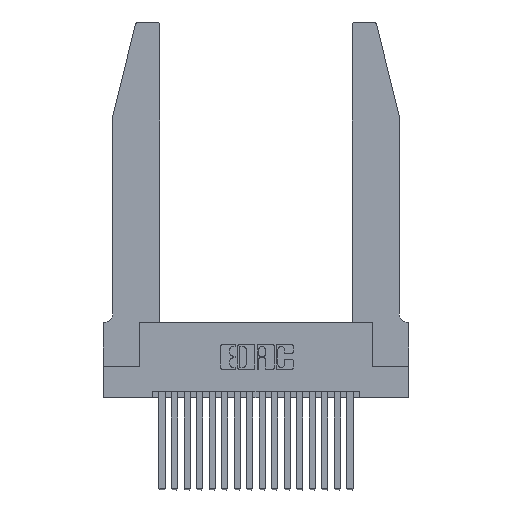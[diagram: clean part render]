
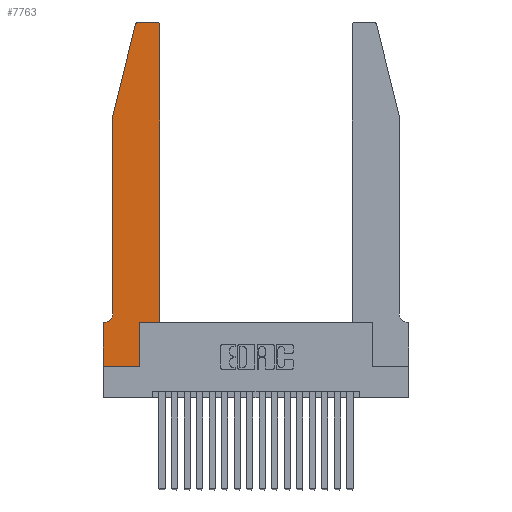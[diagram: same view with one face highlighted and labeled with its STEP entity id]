
A CAD part, top view. The second image highlights one B-rep face of the part: STEP entity #7763.
In plain terms, the highlighted planar face has unit normal (0, 0, 1).
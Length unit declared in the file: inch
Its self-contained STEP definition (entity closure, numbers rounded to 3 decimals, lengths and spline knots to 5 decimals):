
#69 = DIRECTION ( 'NONE',  ( 0., 1., 0. ) ) ;
#285 = ORIENTED_EDGE ( 'NONE', *, *, #6838, .T. ) ;
#444 = DIRECTION ( 'NONE',  ( 1., 0., 0. ) ) ;
#579 = CARTESIAN_POINT ( 'NONE',  ( 0.0755, 2., 0.37 ) ) ;
#1113 = VERTEX_POINT ( 'NONE', #9203 ) ;
#1130 = LINE ( 'NONE', #14866, #9741 ) ;
#1333 = CARTESIAN_POINT ( 'NONE',  ( 0., 0.35, 0.37 ) ) ;
#1350 = CARTESIAN_POINT ( 'NONE',  ( 0.2865, 0.35, 0.37 ) ) ;
#1399 = DIRECTION ( 'NONE',  ( 1., 0., 0. ) ) ;
#1701 = DIRECTION ( 'NONE',  ( 0., 0., 1. ) ) ;
#1765 = FACE_OUTER_BOUND ( 'NONE', #17597, .T. ) ;
#1889 = VERTEX_POINT ( 'NONE', #6471 ) ;
#2112 = DIRECTION ( 'NONE',  ( 0., -1., 0. ) ) ;
#2149 = VERTEX_POINT ( 'NONE', #13323 ) ;
#2468 = CARTESIAN_POINT ( 'NONE',  ( 0.284, 2.75, 0.37 ) ) ;
#2530 = CARTESIAN_POINT ( 'NONE',  ( 0.2865, 0., 0.37 ) ) ;
#2669 = EDGE_CURVE ( 'NONE', #15936, #14158, #4768, .T. ) ;
#2864 = VERTEX_POINT ( 'NONE', #2468 ) ;
#3145 = LINE ( 'NONE', #15876, #6945 ) ;
#3651 = AXIS2_PLACEMENT_3D ( 'NONE', #14541, #5066, #16113 ) ;
#3717 = CIRCLE ( 'NONE', #19159, 0.03 ) ;
#3768 = CARTESIAN_POINT ( 'NONE',  ( 0.0755, 2., 0.37 ) ) ;
#3876 = EDGE_CURVE ( 'NONE', #1113, #12439, #1130, .T. ) ;
#4279 = EDGE_CURVE ( 'NONE', #14158, #1113, #5444, .T. ) ;
#4685 = CARTESIAN_POINT ( 'NONE',  ( 0., 0., 0.37 ) ) ;
#4686 = ORIENTED_EDGE ( 'NONE', *, *, #15532, .T. ) ;
#4768 = LINE ( 'NONE', #1350, #8559 ) ;
#4954 = VECTOR ( 'NONE', #8223, 39.37008 ) ;
#5066 = DIRECTION ( 'NONE',  ( 0., 0., -1. ) ) ;
#5149 = CIRCLE ( 'NONE', #11005, 0.03 ) ;
#5327 = CARTESIAN_POINT ( 'NONE',  ( 0.0755, 2., 0.37 ) ) ;
#5444 = LINE ( 'NONE', #9732, #4954 ) ;
#5517 = VERTEX_POINT ( 'NONE', #1333 ) ;
#5862 = CARTESIAN_POINT ( 'NONE',  ( 0.0755, 0.35, 0.37 ) ) ;
#6303 = CARTESIAN_POINT ( 'NONE',  ( 0.4505, 2.72, 0.37 ) ) ;
#6471 = CARTESIAN_POINT ( 'NONE',  ( 0.4205, 2.75, 0.37 ) ) ;
#6547 = PLANE ( 'NONE',  #8218 ) ;
#6838 = EDGE_CURVE ( 'NONE', #5517, #12768, #9128, .T. ) ;
#6945 = VECTOR ( 'NONE', #17431, 39.37008 ) ;
#7076 = CARTESIAN_POINT ( 'NONE',  ( 0., 0., 0.37 ) ) ;
#7477 = ORIENTED_EDGE ( 'NONE', *, *, #11008, .T. ) ;
#7763 = ADVANCED_FACE ( 'NONE', ( #1765 ), #6547, .T. ) ;
#8180 = CARTESIAN_POINT ( 'NONE',  ( 0., 0.35, 0.37 ) ) ;
#8218 = AXIS2_PLACEMENT_3D ( 'NONE', #8180, #1701, #12889 ) ;
#8223 = DIRECTION ( 'NONE',  ( 1., 0., 0. ) ) ;
#8485 = ORIENTED_EDGE ( 'NONE', *, *, #19275, .T. ) ;
#8559 = VECTOR ( 'NONE', #69, 39.37008 ) ;
#8850 = CARTESIAN_POINT ( 'NONE',  ( 0., 0., 0.37 ) ) ;
#8980 = ORIENTED_EDGE ( 'NONE', *, *, #2669, .T. ) ;
#9128 = LINE ( 'NONE', #8850, #9614 ) ;
#9203 = CARTESIAN_POINT ( 'NONE',  ( 0.4505, 0.35, 0.37 ) ) ;
#9524 = CARTESIAN_POINT ( 'NONE',  ( 0.0055, 0.35, 0.37 ) ) ;
#9614 = VECTOR ( 'NONE', #10420, 39.37008 ) ;
#9732 = CARTESIAN_POINT ( 'NONE',  ( 0.4505, 0.35, 0.37 ) ) ;
#9741 = VECTOR ( 'NONE', #16427, 39.37008 ) ;
#9956 = ORIENTED_EDGE ( 'NONE', *, *, #3876, .T. ) ;
#10088 = LINE ( 'NONE', #5862, #17906 ) ;
#10160 = EDGE_CURVE ( 'NONE', #1889, #2864, #3145, .T. ) ;
#10164 = DIRECTION ( 'NONE',  ( 0., 0., 1. ) ) ;
#10420 = DIRECTION ( 'NONE',  ( 0., -1., 0. ) ) ;
#11005 = AXIS2_PLACEMENT_3D ( 'NONE', #19514, #10164, #444 ) ;
#11008 = EDGE_CURVE ( 'NONE', #2864, #17604, #5149, .T. ) ;
#11042 = VERTEX_POINT ( 'NONE', #3768 ) ;
#11043 = DIRECTION ( 'NONE',  ( 0., 0., 1. ) ) ;
#11228 = VECTOR ( 'NONE', #15692, 39.37008 ) ;
#11651 = ORIENTED_EDGE ( 'NONE', *, *, #14018, .T. ) ;
#12225 = VECTOR ( 'NONE', #16487, 39.37008 ) ;
#12424 = CIRCLE ( 'NONE', #3651, 0.07 ) ;
#12439 = VERTEX_POINT ( 'NONE', #6303 ) ;
#12768 = VERTEX_POINT ( 'NONE', #7076 ) ;
#12889 = DIRECTION ( 'NONE',  ( 1., 0., 0. ) ) ;
#13323 = CARTESIAN_POINT ( 'NONE',  ( 0.0755, 0.42, 0.37 ) ) ;
#13615 = ORIENTED_EDGE ( 'NONE', *, *, #4279, .T. ) ;
#13683 = CARTESIAN_POINT ( 'NONE',  ( 0.2865, 0.35, 0.37 ) ) ;
#14018 = EDGE_CURVE ( 'NONE', #17604, #11042, #16878, .T. ) ;
#14155 = CARTESIAN_POINT ( 'NONE',  ( 0.25487, 2.72718, 0.37 ) ) ;
#14158 = VERTEX_POINT ( 'NONE', #13683 ) ;
#14541 = CARTESIAN_POINT ( 'NONE',  ( 0.0055, 0.42, 0.37 ) ) ;
#14850 = ORIENTED_EDGE ( 'NONE', *, *, #10160, .T. ) ;
#14866 = CARTESIAN_POINT ( 'NONE',  ( 0.4505, 0.35, 0.37 ) ) ;
#14970 = EDGE_CURVE ( 'NONE', #2149, #17009, #12424, .T. ) ;
#15328 = DIRECTION ( 'NONE',  ( -1., 0., 0. ) ) ;
#15498 = EDGE_CURVE ( 'NONE', #12439, #1889, #3717, .T. ) ;
#15532 = EDGE_CURVE ( 'NONE', #12768, #15936, #16360, .T. ) ;
#15692 = DIRECTION ( 'NONE',  ( 1., 0., 0. ) ) ;
#15826 = ORIENTED_EDGE ( 'NONE', *, *, #20531, .T. ) ;
#15876 = CARTESIAN_POINT ( 'NONE',  ( 0.2605, 2.75, 0.37 ) ) ;
#15936 = VERTEX_POINT ( 'NONE', #2530 ) ;
#16113 = DIRECTION ( 'NONE',  ( -1., 0., 0. ) ) ;
#16360 = LINE ( 'NONE', #4685, #11228 ) ;
#16427 = DIRECTION ( 'NONE',  ( 0., 1., 0. ) ) ;
#16487 = DIRECTION ( 'NONE',  ( -0.239, -0.971, 0. ) ) ;
#16878 = LINE ( 'NONE', #579, #12225 ) ;
#17009 = VERTEX_POINT ( 'NONE', #9524 ) ;
#17129 = LINE ( 'NONE', #5327, #20292 ) ;
#17431 = DIRECTION ( 'NONE',  ( -1., 0., 0. ) ) ;
#17597 = EDGE_LOOP ( 'NONE', ( #14850, #7477, #11651, #15826, #20448, #8485, #285, #4686, #8980, #13615, #9956, #18270 ) ) ;
#17604 = VERTEX_POINT ( 'NONE', #14155 ) ;
#17906 = VECTOR ( 'NONE', #15328, 39.37008 ) ;
#18270 = ORIENTED_EDGE ( 'NONE', *, *, #15498, .T. ) ;
#19159 = AXIS2_PLACEMENT_3D ( 'NONE', #20378, #11043, #1399 ) ;
#19275 = EDGE_CURVE ( 'NONE', #17009, #5517, #10088, .T. ) ;
#19514 = CARTESIAN_POINT ( 'NONE',  ( 0.284, 2.72, 0.37 ) ) ;
#20292 = VECTOR ( 'NONE', #2112, 39.37008 ) ;
#20378 = CARTESIAN_POINT ( 'NONE',  ( 0.4205, 2.72, 0.37 ) ) ;
#20448 = ORIENTED_EDGE ( 'NONE', *, *, #14970, .T. ) ;
#20531 = EDGE_CURVE ( 'NONE', #11042, #2149, #17129, .T. ) ;
